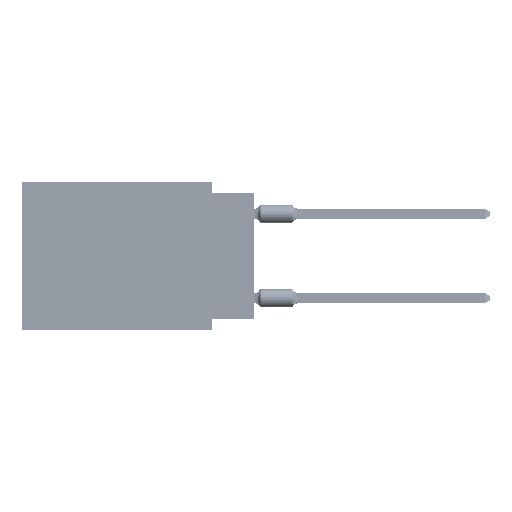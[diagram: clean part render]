
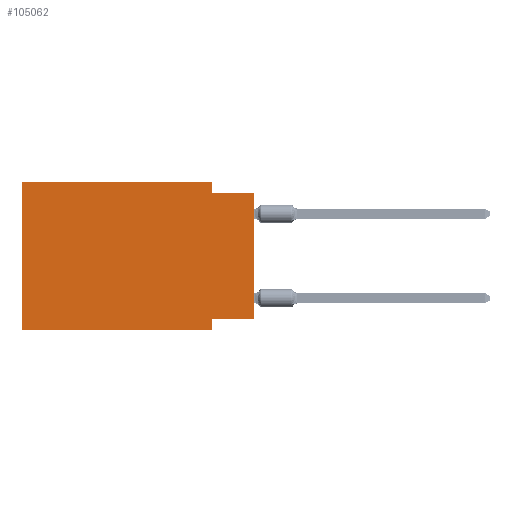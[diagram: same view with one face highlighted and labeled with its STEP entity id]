
A CAD part, left-side view. The second image highlights one B-rep face of the part: STEP entity #105062.
In plain terms, the highlighted planar face has unit normal (-1, 0, 0).
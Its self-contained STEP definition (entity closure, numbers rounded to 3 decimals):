
#1636 = EDGE_CURVE ( 'NONE', #49835, #53608, #11846, .T. ) ;
#5317 = DIRECTION ( 'NONE',  ( 0., 0., 1. ) ) ;
#7989 = LINE ( 'NONE', #88135, #70294 ) ;
#11846 = LINE ( 'NONE', #47037, #87314 ) ;
#14306 = LINE ( 'NONE', #111168, #70418 ) ;
#14489 = CARTESIAN_POINT ( 'NONE',  ( 0., 0., 0. ) ) ;
#18523 = VERTEX_POINT ( 'NONE', #104100 ) ;
#19022 = EDGE_LOOP ( 'NONE', ( #85591, #19280, #23866, #84076, #44341, #97270, #40952, #70456 ) ) ;
#19280 = ORIENTED_EDGE ( 'NONE', *, *, #68872, .F. ) ;
#23556 = DIRECTION ( 'NONE',  ( 1., 0., 0. ) ) ;
#23616 = VERTEX_POINT ( 'NONE', #81030 ) ;
#23731 = VECTOR ( 'NONE', #100422, 1000. ) ;
#23866 = ORIENTED_EDGE ( 'NONE', *, *, #104534, .F. ) ;
#24018 = CARTESIAN_POINT ( 'NONE',  ( 0., 13.97, -8.89 ) ) ;
#24223 = EDGE_CURVE ( 'NONE', #72997, #23616, #7989, .T. ) ;
#24849 = LINE ( 'NONE', #110799, #59190 ) ;
#25708 = AXIS2_PLACEMENT_3D ( 'NONE', #102551, #23556, #58729 ) ;
#27311 = CARTESIAN_POINT ( 'NONE',  ( 0., 2.54, -8.255 ) ) ;
#32196 = FACE_OUTER_BOUND ( 'NONE', #19022, .T. ) ;
#35375 = VECTOR ( 'NONE', #111931, 1000. ) ;
#39042 = VECTOR ( 'NONE', #88465, 1000. ) ;
#40952 = ORIENTED_EDGE ( 'NONE', *, *, #24223, .F. ) ;
#42360 = LINE ( 'NONE', #95981, #39042 ) ;
#44341 = ORIENTED_EDGE ( 'NONE', *, *, #1636, .F. ) ;
#47037 = CARTESIAN_POINT ( 'NONE',  ( 0., 13.97, 0. ) ) ;
#49835 = VERTEX_POINT ( 'NONE', #24018 ) ;
#53608 = VERTEX_POINT ( 'NONE', #104578 ) ;
#54739 = CARTESIAN_POINT ( 'NONE',  ( 0., 2.54, -0.635 ) ) ;
#55595 = EDGE_CURVE ( 'NONE', #107488, #72997, #24849, .T. ) ;
#57205 = CARTESIAN_POINT ( 'NONE',  ( 0., 0., -8.255 ) ) ;
#57551 = LINE ( 'NONE', #91022, #108150 ) ;
#58729 = DIRECTION ( 'NONE',  ( 0., 0., -1. ) ) ;
#59190 = VECTOR ( 'NONE', #76177, 1000. ) ;
#67365 = PLANE ( 'NONE',  #25708 ) ;
#68186 = CARTESIAN_POINT ( 'NONE',  ( 0., 2.54, 0. ) ) ;
#68872 = EDGE_CURVE ( 'NONE', #85635, #18523, #42360, .T. ) ;
#70294 = VECTOR ( 'NONE', #87559, 1000. ) ;
#70418 = VECTOR ( 'NONE', #74302, 1000. ) ;
#70456 = ORIENTED_EDGE ( 'NONE', *, *, #55595, .F. ) ;
#72997 = VERTEX_POINT ( 'NONE', #27311 ) ;
#73886 = LINE ( 'NONE', #109067, #23731 ) ;
#74302 = DIRECTION ( 'NONE',  ( 0., -1., 0. ) ) ;
#75706 = VERTEX_POINT ( 'NONE', #68186 ) ;
#76177 = DIRECTION ( 'NONE',  ( 0., 1., 0. ) ) ;
#81030 = CARTESIAN_POINT ( 'NONE',  ( 0., 2.54, -8.89 ) ) ;
#83670 = EDGE_CURVE ( 'NONE', #49835, #23616, #57551, .T. ) ;
#84052 = DIRECTION ( 'NONE',  ( 0., -1., 0. ) ) ;
#84076 = ORIENTED_EDGE ( 'NONE', *, *, #113694, .F. ) ;
#85591 = ORIENTED_EDGE ( 'NONE', *, *, #108328, .T. ) ;
#85635 = VERTEX_POINT ( 'NONE', #54739 ) ;
#86552 = LINE ( 'NONE', #14489, #35375 ) ;
#87314 = VECTOR ( 'NONE', #5317, 1000. ) ;
#87559 = DIRECTION ( 'NONE',  ( 0., 0., -1. ) ) ;
#88135 = CARTESIAN_POINT ( 'NONE',  ( 0., 2.54, -8.89 ) ) ;
#88465 = DIRECTION ( 'NONE',  ( 0., -1., 0. ) ) ;
#91022 = CARTESIAN_POINT ( 'NONE',  ( 0., 13.97, -8.89 ) ) ;
#95981 = CARTESIAN_POINT ( 'NONE',  ( 0., 0., -0.635 ) ) ;
#97270 = ORIENTED_EDGE ( 'NONE', *, *, #83670, .T. ) ;
#100422 = DIRECTION ( 'NONE',  ( 0., 0., -1. ) ) ;
#102551 = CARTESIAN_POINT ( 'NONE',  ( 0., 13.97, 0. ) ) ;
#104100 = CARTESIAN_POINT ( 'NONE',  ( 0., 0., -0.635 ) ) ;
#104534 = EDGE_CURVE ( 'NONE', #75706, #85635, #73886, .T. ) ;
#104578 = CARTESIAN_POINT ( 'NONE',  ( 0., 13.97, 0. ) ) ;
#105062 = ADVANCED_FACE ( 'NONE', ( #32196 ), #67365, .F. ) ;
#107488 = VERTEX_POINT ( 'NONE', #57205 ) ;
#108150 = VECTOR ( 'NONE', #84052, 1000. ) ;
#108328 = EDGE_CURVE ( 'NONE', #107488, #18523, #86552, .T. ) ;
#109067 = CARTESIAN_POINT ( 'NONE',  ( 0., 2.54, 0. ) ) ;
#110799 = CARTESIAN_POINT ( 'NONE',  ( 0., 0., -8.255 ) ) ;
#111168 = CARTESIAN_POINT ( 'NONE',  ( 0., 13.97, 0. ) ) ;
#111931 = DIRECTION ( 'NONE',  ( 0., 0., 1. ) ) ;
#113694 = EDGE_CURVE ( 'NONE', #53608, #75706, #14306, .T. ) ;
